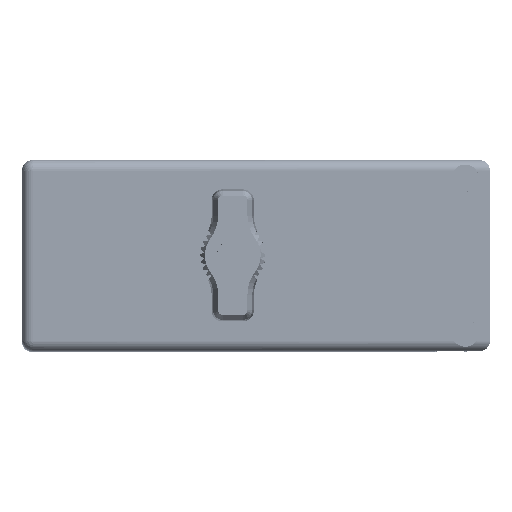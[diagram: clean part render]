
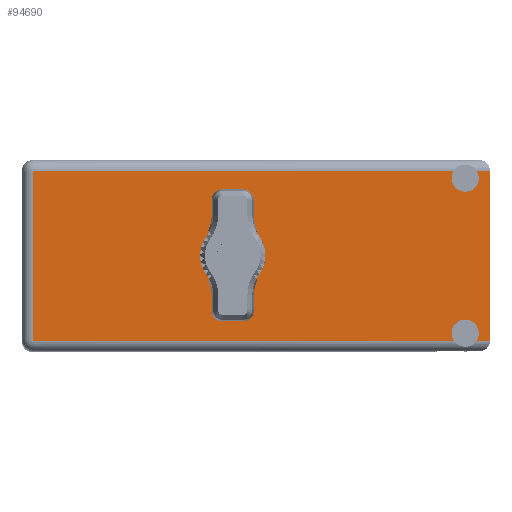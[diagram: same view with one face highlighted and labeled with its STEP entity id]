
A CAD part, top view. The second image highlights one B-rep face of the part: STEP entity #94690.
In plain terms, the highlighted face is planar.
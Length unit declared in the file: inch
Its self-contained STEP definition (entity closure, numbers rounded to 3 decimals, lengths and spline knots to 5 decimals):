
#101 = ORIENTED_EDGE ( 'NONE', *, *, #69671, .F. ) ;
#1235 = DIRECTION ( 'NONE',  ( 0., 1., 0. ) ) ;
#3021 = ORIENTED_EDGE ( 'NONE', *, *, #33974, .F. ) ;
#4190 = CARTESIAN_POINT ( 'NONE',  ( -1.359, 1.675, -0.617 ) ) ;
#4959 = VERTEX_POINT ( 'NONE', #83080 ) ;
#8723 = DIRECTION ( 'NONE',  ( 0., 0., 1. ) ) ;
#10148 = AXIS2_PLACEMENT_3D ( 'NONE', #4190, #94383, #18895 ) ;
#13230 = CIRCLE ( 'NONE', #43764, 0.125 ) ;
#14389 = ORIENTED_EDGE ( 'NONE', *, *, #18629, .T. ) ;
#15159 = AXIS2_PLACEMENT_3D ( 'NONE', #37595, #30786, #89928 ) ;
#15946 = CARTESIAN_POINT ( 'NONE',  ( 1.499, 1.675, 0.5 ) ) ;
#16341 = ORIENTED_EDGE ( 'NONE', *, *, #53323, .F. ) ;
#17520 = DIRECTION ( 'NONE',  ( 0., 0., 1. ) ) ;
#18629 = EDGE_CURVE ( 'NONE', #51247, #94845, #29412, .T. ) ;
#18721 = VECTOR ( 'NONE', #64924, 39.37008 ) ;
#18895 = DIRECTION ( 'NONE',  ( -1., 0., 0. ) ) ;
#20096 = VERTEX_POINT ( 'NONE', #24830 ) ;
#20791 = CARTESIAN_POINT ( 'NONE',  ( 1.57281, 1.675, 0.547 ) ) ;
#20798 = CARTESIAN_POINT ( 'NONE',  ( -1.359, 1.675, -0.547 ) ) ;
#21348 = EDGE_CURVE ( 'NONE', #33713, #4959, #51590, .T. ) ;
#22643 = CARTESIAN_POINT ( 'NONE',  ( -1.289, 1.675, 0.547 ) ) ;
#23322 = EDGE_CURVE ( 'NONE', #88360, #51247, #96846, .T. ) ;
#24360 = DIRECTION ( 'NONE',  ( 0., 1., 0. ) ) ;
#24830 = CARTESIAN_POINT ( 'NONE',  ( 1.499, 1.675, -0.4125 ) ) ;
#26451 = ORIENTED_EDGE ( 'NONE', *, *, #53589, .F. ) ;
#29139 = DIRECTION ( 'NONE',  ( 0., 0., 1. ) ) ;
#29201 = CIRCLE ( 'NONE', #15159, 0.125 ) ;
#29412 = LINE ( 'NONE', #41738, #39849 ) ;
#30393 = ORIENTED_EDGE ( 'NONE', *, *, #59631, .F. ) ;
#30786 = DIRECTION ( 'NONE',  ( 0., 1., 0. ) ) ;
#31727 = VERTEX_POINT ( 'NONE', #63988 ) ;
#31735 = ORIENTED_EDGE ( 'NONE', *, *, #54148, .T. ) ;
#33713 = VERTEX_POINT ( 'NONE', #58083 ) ;
#33829 = PLANE ( 'NONE',  #10148 ) ;
#33974 = EDGE_CURVE ( 'NONE', #63468, #33713, #60234, .T. ) ;
#34484 = CARTESIAN_POINT ( 'NONE',  ( 1.42519, 1.675, -0.547 ) ) ;
#34571 = DIRECTION ( 'NONE',  ( 0., 0., 1. ) ) ;
#37595 = CARTESIAN_POINT ( 'NONE',  ( 0., 1.675, 0. ) ) ;
#38907 = DIRECTION ( 'NONE',  ( -1., 0., 0. ) ) ;
#39018 = CARTESIAN_POINT ( 'NONE',  ( 1.499, 1.675, 0.5 ) ) ;
#39849 = VECTOR ( 'NONE', #17520, 39.37008 ) ;
#39923 = CARTESIAN_POINT ( 'NONE',  ( 1.659, 1.675, -0.547 ) ) ;
#41239 = VECTOR ( 'NONE', #91937, 39.37008 ) ;
#41488 = CARTESIAN_POINT ( 'NONE',  ( -1.289, 1.675, -0.547 ) ) ;
#41738 = CARTESIAN_POINT ( 'NONE',  ( -1.289, 1.675, -0.617 ) ) ;
#42259 = LINE ( 'NONE', #95402, #63321 ) ;
#42847 = CARTESIAN_POINT ( 'NONE',  ( 0., 1.675, 0. ) ) ;
#43764 = AXIS2_PLACEMENT_3D ( 'NONE', #42847, #96138, #29139 ) ;
#44893 = DIRECTION ( 'NONE',  ( 0., 0., 1. ) ) ;
#45627 = DIRECTION ( 'NONE',  ( 0., 0., 1. ) ) ;
#46671 = AXIS2_PLACEMENT_3D ( 'NONE', #82187, #89672, #44893 ) ;
#46772 = EDGE_CURVE ( 'NONE', #75787, #93110, #87669, .T. ) ;
#47137 = CARTESIAN_POINT ( 'NONE',  ( -1.359, 1.675, -0.547 ) ) ;
#51247 = VERTEX_POINT ( 'NONE', #41488 ) ;
#51590 = CIRCLE ( 'NONE', #95979, 0.0875 ) ;
#53323 = EDGE_CURVE ( 'NONE', #75787, #31727, #84477, .T. ) ;
#53589 = EDGE_CURVE ( 'NONE', #65792, #63875, #13230, .T. ) ;
#54148 = EDGE_CURVE ( 'NONE', #94845, #4959, #42259, .T. ) ;
#56592 = EDGE_LOOP ( 'NONE', ( #26451, #95587 ) ) ;
#58083 = CARTESIAN_POINT ( 'NONE',  ( 1.499, 1.675, 0.4125 ) ) ;
#59631 = EDGE_CURVE ( 'NONE', #20096, #93110, #71012, .T. ) ;
#60234 = CIRCLE ( 'NONE', #71155, 0.0875 ) ;
#63321 = VECTOR ( 'NONE', #94094, 39.37008 ) ;
#63468 = VERTEX_POINT ( 'NONE', #20791 ) ;
#63875 = VERTEX_POINT ( 'NONE', #71010 ) ;
#63988 = CARTESIAN_POINT ( 'NONE',  ( 1.659, 1.675, 0.547 ) ) ;
#64407 = DIRECTION ( 'NONE',  ( 0., 1., 0. ) ) ;
#64707 = ORIENTED_EDGE ( 'NONE', *, *, #95802, .T. ) ;
#64924 = DIRECTION ( 'NONE',  ( -1., 0., 0. ) ) ;
#65792 = VERTEX_POINT ( 'NONE', #78257 ) ;
#66243 = VECTOR ( 'NONE', #83115, 39.37008 ) ;
#67424 = CARTESIAN_POINT ( 'NONE',  ( 1.659, 1.675, 0.547 ) ) ;
#69671 = EDGE_CURVE ( 'NONE', #88360, #20096, #75907, .T. ) ;
#70675 = CARTESIAN_POINT ( 'NONE',  ( 1.659, 1.675, 0.617 ) ) ;
#71010 = CARTESIAN_POINT ( 'NONE',  ( 0., 1.675, -0.125 ) ) ;
#71012 = CIRCLE ( 'NONE', #93019, 0.0875 ) ;
#71155 = AXIS2_PLACEMENT_3D ( 'NONE', #39018, #1235, #8723 ) ;
#71409 = EDGE_LOOP ( 'NONE', ( #31735, #89011, #3021, #64707, #16341, #86826, #30393, #101, #82686, #14389 ) ) ;
#75787 = VERTEX_POINT ( 'NONE', #39923 ) ;
#75843 = VECTOR ( 'NONE', #38907, 39.37008 ) ;
#75907 = CIRCLE ( 'NONE', #46671, 0.0875 ) ;
#78257 = CARTESIAN_POINT ( 'NONE',  ( 0., 1.675, 0.125 ) ) ;
#78807 = CARTESIAN_POINT ( 'NONE',  ( 1.499, 1.675, -0.5 ) ) ;
#79695 = CARTESIAN_POINT ( 'NONE',  ( 1.57281, 1.675, -0.547 ) ) ;
#80524 = FACE_BOUND ( 'NONE', #56592, .T. ) ;
#81438 = LINE ( 'NONE', #67424, #66243 ) ;
#82187 = CARTESIAN_POINT ( 'NONE',  ( 1.499, 1.675, -0.5 ) ) ;
#82686 = ORIENTED_EDGE ( 'NONE', *, *, #23322, .T. ) ;
#83080 = CARTESIAN_POINT ( 'NONE',  ( 1.42519, 1.675, 0.547 ) ) ;
#83115 = DIRECTION ( 'NONE',  ( 1., 0., 0. ) ) ;
#84477 = LINE ( 'NONE', #70675, #41239 ) ;
#86826 = ORIENTED_EDGE ( 'NONE', *, *, #46772, .T. ) ;
#87669 = LINE ( 'NONE', #20798, #18721 ) ;
#88360 = VERTEX_POINT ( 'NONE', #34484 ) ;
#89011 = ORIENTED_EDGE ( 'NONE', *, *, #21348, .F. ) ;
#89672 = DIRECTION ( 'NONE',  ( 0., 1., 0. ) ) ;
#89928 = DIRECTION ( 'NONE',  ( 0., 0., 1. ) ) ;
#90973 = FACE_OUTER_BOUND ( 'NONE', #71409, .T. ) ;
#91937 = DIRECTION ( 'NONE',  ( 0., 0., 1. ) ) ;
#93019 = AXIS2_PLACEMENT_3D ( 'NONE', #78807, #64407, #34571 ) ;
#93110 = VERTEX_POINT ( 'NONE', #79695 ) ;
#93748 = EDGE_CURVE ( 'NONE', #63875, #65792, #29201, .T. ) ;
#94094 = DIRECTION ( 'NONE',  ( 1., 0., 0. ) ) ;
#94383 = DIRECTION ( 'NONE',  ( 0., 1., 0. ) ) ;
#94690 = ADVANCED_FACE ( 'NONE', ( #80524, #90973 ), #33829, .T. ) ;
#94845 = VERTEX_POINT ( 'NONE', #22643 ) ;
#95402 = CARTESIAN_POINT ( 'NONE',  ( 1.659, 1.675, 0.547 ) ) ;
#95587 = ORIENTED_EDGE ( 'NONE', *, *, #93748, .F. ) ;
#95802 = EDGE_CURVE ( 'NONE', #63468, #31727, #81438, .T. ) ;
#95979 = AXIS2_PLACEMENT_3D ( 'NONE', #15946, #24360, #45627 ) ;
#96138 = DIRECTION ( 'NONE',  ( 0., 1., 0. ) ) ;
#96846 = LINE ( 'NONE', #47137, #75843 ) ;
